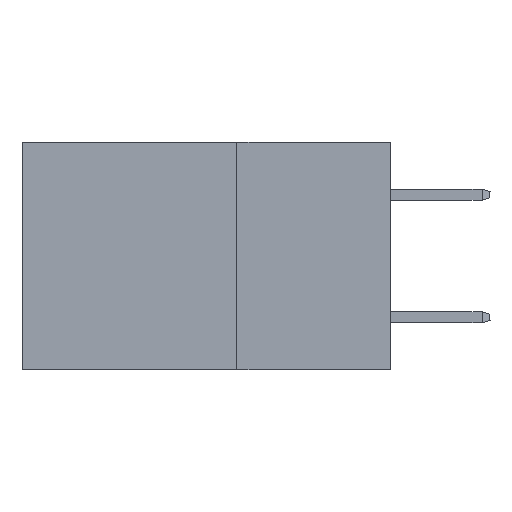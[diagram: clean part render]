
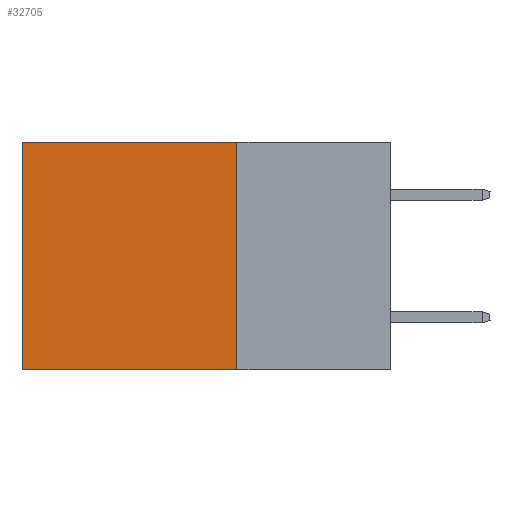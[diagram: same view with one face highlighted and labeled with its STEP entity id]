
A CAD part, left-side view. The second image highlights one B-rep face of the part: STEP entity #32705.
In plain terms, the highlighted planar face has unit normal (-1, 0, 0).
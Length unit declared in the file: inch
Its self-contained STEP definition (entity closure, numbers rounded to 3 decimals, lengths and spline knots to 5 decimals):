
#848 = VECTOR ( 'NONE', #17293, 39.37008 ) ;
#3614 = EDGE_CURVE ( 'NONE', #25124, #6019, #6464, .T. ) ;
#4103 = ORIENTED_EDGE ( 'NONE', *, *, #3614, .T. ) ;
#4413 = ORIENTED_EDGE ( 'NONE', *, *, #22268, .F. ) ;
#5557 = CARTESIAN_POINT ( 'NONE',  ( 0.2875, 0.25, 0. ) ) ;
#6019 = VERTEX_POINT ( 'NONE', #19787 ) ;
#6334 = ORIENTED_EDGE ( 'NONE', *, *, #24996, .F. ) ;
#6464 = LINE ( 'NONE', #13028, #13144 ) ;
#7560 = AXIS2_PLACEMENT_3D ( 'NONE', #25793, #31865, #31736 ) ;
#11730 = VERTEX_POINT ( 'NONE', #5557 ) ;
#12846 = CARTESIAN_POINT ( 'NONE',  ( 0.2875, 0.6, 0. ) ) ;
#13028 = CARTESIAN_POINT ( 'NONE',  ( 0.2875, 0.6, 0. ) ) ;
#13144 = VECTOR ( 'NONE', #18613, 39.37008 ) ;
#13402 = VECTOR ( 'NONE', #33393, 39.37008 ) ;
#14234 = CARTESIAN_POINT ( 'NONE',  ( 0.2875, 0.25, 0. ) ) ;
#17293 = DIRECTION ( 'NONE',  ( 0., 1., 0. ) ) ;
#18613 = DIRECTION ( 'NONE',  ( 0., 0., -1. ) ) ;
#18960 = DIRECTION ( 'NONE',  ( 0., 0., -1. ) ) ;
#19787 = CARTESIAN_POINT ( 'NONE',  ( 0.2875, 0.6, -0.37 ) ) ;
#22268 = EDGE_CURVE ( 'NONE', #26388, #6019, #38827, .T. ) ;
#23982 = FACE_OUTER_BOUND ( 'NONE', #35419, .T. ) ;
#24996 = EDGE_CURVE ( 'NONE', #11730, #26388, #26627, .T. ) ;
#25124 = VERTEX_POINT ( 'NONE', #12846 ) ;
#25793 = CARTESIAN_POINT ( 'NONE',  ( 0.2875, 0.25, 0. ) ) ;
#26388 = VERTEX_POINT ( 'NONE', #30614 ) ;
#26627 = LINE ( 'NONE', #31392, #33810 ) ;
#29947 = LINE ( 'NONE', #14234, #848 ) ;
#30614 = CARTESIAN_POINT ( 'NONE',  ( 0.2875, 0.25, -0.37 ) ) ;
#31392 = CARTESIAN_POINT ( 'NONE',  ( 0.2875, 0.25, 0. ) ) ;
#31736 = DIRECTION ( 'NONE',  ( 0., 0., -1. ) ) ;
#31865 = DIRECTION ( 'NONE',  ( 1., 0., 0. ) ) ;
#32068 = ORIENTED_EDGE ( 'NONE', *, *, #36770, .T. ) ;
#32705 = ADVANCED_FACE ( 'NONE', ( #23982 ), #34657, .F. ) ;
#33393 = DIRECTION ( 'NONE',  ( 0., 1., 0. ) ) ;
#33810 = VECTOR ( 'NONE', #18960, 39.37008 ) ;
#34657 = PLANE ( 'NONE',  #7560 ) ;
#35419 = EDGE_LOOP ( 'NONE', ( #4103, #4413, #6334, #32068 ) ) ;
#36349 = CARTESIAN_POINT ( 'NONE',  ( 0.2875, 0.25, -0.37 ) ) ;
#36770 = EDGE_CURVE ( 'NONE', #11730, #25124, #29947, .T. ) ;
#38827 = LINE ( 'NONE', #36349, #13402 ) ;
